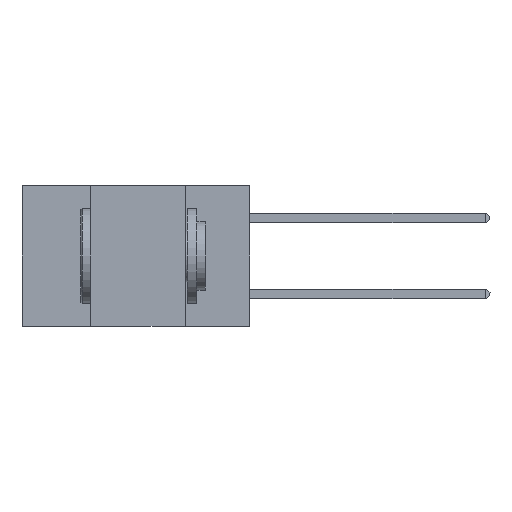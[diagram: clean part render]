
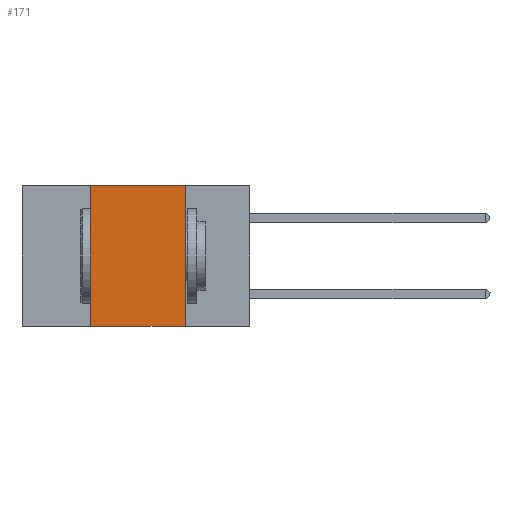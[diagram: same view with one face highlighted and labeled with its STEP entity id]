
A CAD part, left-side view. The second image highlights one B-rep face of the part: STEP entity #171.
In plain terms, the highlighted planar face has unit normal (-1, 0, 0).
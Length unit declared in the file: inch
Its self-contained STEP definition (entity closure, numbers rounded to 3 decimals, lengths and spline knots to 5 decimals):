
#171 = ADVANCED_FACE ( 'NONE', ( #5544 ), #7940, .F. ) ;
#329 = EDGE_CURVE ( 'NONE', #3469, #922, #10581, .T. ) ;
#905 = CARTESIAN_POINT ( 'NONE',  ( 0., 0.17, 0. ) ) ;
#922 = VERTEX_POINT ( 'NONE', #4457 ) ;
#931 = CARTESIAN_POINT ( 'NONE',  ( 0., 0.6, 0. ) ) ;
#1397 = LINE ( 'NONE', #6536, #2345 ) ;
#1846 = ORIENTED_EDGE ( 'NONE', *, *, #329, .T. ) ;
#2230 = VERTEX_POINT ( 'NONE', #905 ) ;
#2345 = VECTOR ( 'NONE', #9863, 39.37008 ) ;
#2375 = CARTESIAN_POINT ( 'NONE',  ( 0., 0.17, 0. ) ) ;
#3290 = LINE ( 'NONE', #931, #5273 ) ;
#3469 = VERTEX_POINT ( 'NONE', #10324 ) ;
#3555 = AXIS2_PLACEMENT_3D ( 'NONE', #6126, #10388, #8693 ) ;
#3566 = CARTESIAN_POINT ( 'NONE',  ( 0., 0.6, -0.37 ) ) ;
#4457 = CARTESIAN_POINT ( 'NONE',  ( 0., 0.17, -0.37 ) ) ;
#4838 = VERTEX_POINT ( 'NONE', #9830 ) ;
#4990 = ORIENTED_EDGE ( 'NONE', *, *, #8291, .F. ) ;
#5273 = VECTOR ( 'NONE', #6852, 39.37008 ) ;
#5334 = DIRECTION ( 'NONE',  ( 0., -1., 0. ) ) ;
#5544 = FACE_OUTER_BOUND ( 'NONE', #6883, .T. ) ;
#6072 = VECTOR ( 'NONE', #5334, 39.37008 ) ;
#6126 = CARTESIAN_POINT ( 'NONE',  ( 0., 0.6, 0. ) ) ;
#6536 = CARTESIAN_POINT ( 'NONE',  ( 0., 0.42, 0. ) ) ;
#6838 = VECTOR ( 'NONE', #10739, 39.37008 ) ;
#6852 = DIRECTION ( 'NONE',  ( 0., -1., 0. ) ) ;
#6883 = EDGE_LOOP ( 'NONE', ( #9464, #9031, #4990, #1846 ) ) ;
#7940 = PLANE ( 'NONE',  #3555 ) ;
#8291 = EDGE_CURVE ( 'NONE', #3469, #4838, #1397, .T. ) ;
#8630 = EDGE_CURVE ( 'NONE', #4838, #2230, #3290, .T. ) ;
#8693 = DIRECTION ( 'NONE',  ( 0., 0., -1. ) ) ;
#9031 = ORIENTED_EDGE ( 'NONE', *, *, #8630, .F. ) ;
#9070 = LINE ( 'NONE', #2375, #6838 ) ;
#9439 = EDGE_CURVE ( 'NONE', #2230, #922, #9070, .T. ) ;
#9464 = ORIENTED_EDGE ( 'NONE', *, *, #9439, .F. ) ;
#9830 = CARTESIAN_POINT ( 'NONE',  ( 0., 0.42, 0. ) ) ;
#9863 = DIRECTION ( 'NONE',  ( 0., 0., 1. ) ) ;
#10324 = CARTESIAN_POINT ( 'NONE',  ( 0., 0.42, -0.37 ) ) ;
#10388 = DIRECTION ( 'NONE',  ( 1., 0., 0. ) ) ;
#10581 = LINE ( 'NONE', #3566, #6072 ) ;
#10739 = DIRECTION ( 'NONE',  ( 0., 0., -1. ) ) ;
